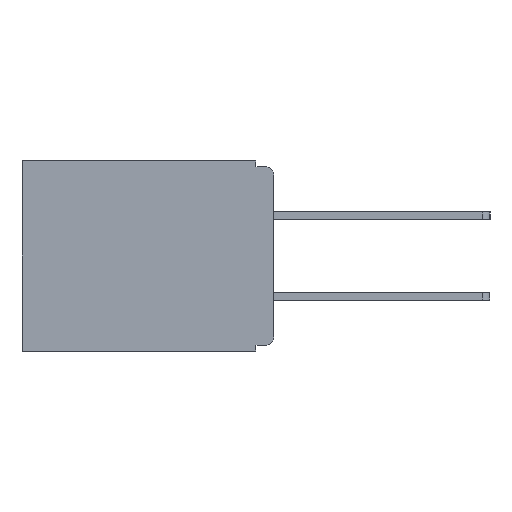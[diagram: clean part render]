
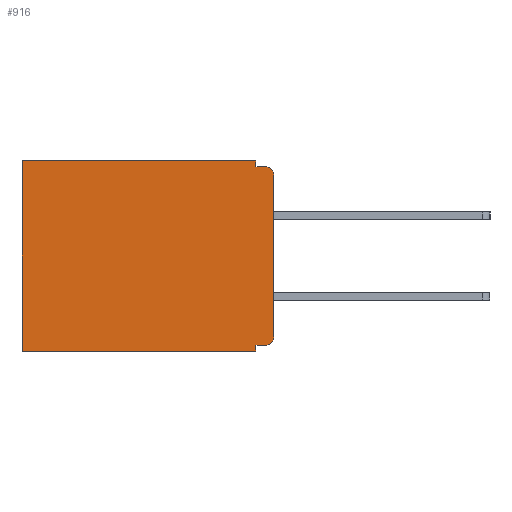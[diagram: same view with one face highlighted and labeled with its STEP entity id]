
A CAD part, left-side view. The second image highlights one B-rep face of the part: STEP entity #916.
In plain terms, the highlighted planar face has unit normal (-1, 0, 0).
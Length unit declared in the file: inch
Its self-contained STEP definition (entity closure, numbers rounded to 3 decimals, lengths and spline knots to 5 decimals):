
#257 = EDGE_CURVE ( 'NONE', #17547, #11450, #16624, .T. ) ;
#295 = CARTESIAN_POINT ( 'NONE',  ( 0.3, 0., -0.305 ) ) ;
#729 = EDGE_CURVE ( 'NONE', #16761, #9705, #21388, .T. ) ;
#916 = ADVANCED_FACE ( 'NONE', ( #12551 ), #16678, .F. ) ;
#1194 = DIRECTION ( 'NONE',  ( 1., 0., 0. ) ) ;
#1379 = EDGE_CURVE ( 'NONE', #1905, #20736, #11943, .T. ) ;
#1408 = LINE ( 'NONE', #9145, #15512 ) ;
#1905 = VERTEX_POINT ( 'NONE', #21565 ) ;
#1926 = VERTEX_POINT ( 'NONE', #21072 ) ;
#1975 = VECTOR ( 'NONE', #15473, 39.37008 ) ;
#2044 = VERTEX_POINT ( 'NONE', #295 ) ;
#2664 = CIRCLE ( 'NONE', #19010, 0.015 ) ;
#3220 = ORIENTED_EDGE ( 'NONE', *, *, #19038, .T. ) ;
#3266 = VECTOR ( 'NONE', #14020, 39.37008 ) ;
#3388 = DIRECTION ( 'NONE',  ( 0., 0., -1. ) ) ;
#5273 = ORIENTED_EDGE ( 'NONE', *, *, #23190, .T. ) ;
#6233 = CARTESIAN_POINT ( 'NONE',  ( 0.3, 0., -0.025 ) ) ;
#6611 = ORIENTED_EDGE ( 'NONE', *, *, #7758, .F. ) ;
#6916 = VECTOR ( 'NONE', #12707, 39.37008 ) ;
#7016 = CARTESIAN_POINT ( 'NONE',  ( 0.3, 0.031, -0.33 ) ) ;
#7121 = CARTESIAN_POINT ( 'NONE',  ( 0.3, 0.031, -0.32 ) ) ;
#7141 = CARTESIAN_POINT ( 'NONE',  ( 0.3, 0., -0.33 ) ) ;
#7564 = CARTESIAN_POINT ( 'NONE',  ( 0.3, 0., -0.33 ) ) ;
#7758 = EDGE_CURVE ( 'NONE', #20229, #9705, #18964, .T. ) ;
#8225 = CARTESIAN_POINT ( 'NONE',  ( 0.3, 0.015, -0.025 ) ) ;
#8799 = EDGE_CURVE ( 'NONE', #11450, #1926, #1408, .T. ) ;
#8813 = DIRECTION ( 'NONE',  ( 0., 0., -1. ) ) ;
#8889 = ORIENTED_EDGE ( 'NONE', *, *, #1379, .F. ) ;
#9055 = VERTEX_POINT ( 'NONE', #6233 ) ;
#9145 = CARTESIAN_POINT ( 'NONE',  ( 0.3, 0., -0.01 ) ) ;
#9475 = CARTESIAN_POINT ( 'NONE',  ( 0.3, 0.015, -0.305 ) ) ;
#9705 = VERTEX_POINT ( 'NONE', #13514 ) ;
#9715 = LINE ( 'NONE', #7016, #14582 ) ;
#10047 = DIRECTION ( 'NONE',  ( 0., 0., -1. ) ) ;
#10488 = CARTESIAN_POINT ( 'NONE',  ( 0.3, 0.437, -0.33 ) ) ;
#10708 = CARTESIAN_POINT ( 'NONE',  ( 0.3, 0., -0.33 ) ) ;
#11182 = CARTESIAN_POINT ( 'NONE',  ( 0.3, 0.031, 0. ) ) ;
#11273 = DIRECTION ( 'NONE',  ( 0., 0., -1. ) ) ;
#11450 = VERTEX_POINT ( 'NONE', #22516 ) ;
#11943 = LINE ( 'NONE', #19986, #16837 ) ;
#12072 = CARTESIAN_POINT ( 'NONE',  ( 0.3, 0., 0. ) ) ;
#12343 = ORIENTED_EDGE ( 'NONE', *, *, #257, .F. ) ;
#12551 = FACE_OUTER_BOUND ( 'NONE', #17389, .T. ) ;
#12707 = DIRECTION ( 'NONE',  ( 0., 0., -1. ) ) ;
#12970 = ORIENTED_EDGE ( 'NONE', *, *, #22609, .T. ) ;
#13514 = CARTESIAN_POINT ( 'NONE',  ( 0.3, 0.437, -0.33 ) ) ;
#13988 = CARTESIAN_POINT ( 'NONE',  ( 0.3, 0.031, 0. ) ) ;
#14020 = DIRECTION ( 'NONE',  ( 0., 1., 0. ) ) ;
#14120 = VECTOR ( 'NONE', #22031, 39.37008 ) ;
#14582 = VECTOR ( 'NONE', #8813, 39.37008 ) ;
#14674 = DIRECTION ( 'NONE',  ( 0., -1., 0. ) ) ;
#14936 = CARTESIAN_POINT ( 'NONE',  ( 0.3, 0.031, -0.33 ) ) ;
#15131 = CIRCLE ( 'NONE', #22781, 0.015 ) ;
#15473 = DIRECTION ( 'NONE',  ( 0., 0., -1. ) ) ;
#15512 = VECTOR ( 'NONE', #14674, 39.37008 ) ;
#15658 = LINE ( 'NONE', #10708, #19895 ) ;
#16264 = CARTESIAN_POINT ( 'NONE',  ( 0.3, 0.437, 0. ) ) ;
#16624 = LINE ( 'NONE', #13988, #1975 ) ;
#16678 = PLANE ( 'NONE',  #21882 ) ;
#16761 = VERTEX_POINT ( 'NONE', #16264 ) ;
#16837 = VECTOR ( 'NONE', #19875, 39.37008 ) ;
#17375 = EDGE_CURVE ( 'NONE', #9055, #2044, #15658, .T. ) ;
#17389 = EDGE_LOOP ( 'NONE', ( #21274, #12970, #17854, #12343, #5273, #21828, #6611, #18750, #8889, #3220 ) ) ;
#17547 = VERTEX_POINT ( 'NONE', #11182 ) ;
#17854 = ORIENTED_EDGE ( 'NONE', *, *, #8799, .F. ) ;
#18750 = ORIENTED_EDGE ( 'NONE', *, *, #21571, .F. ) ;
#18964 = LINE ( 'NONE', #7564, #14120 ) ;
#19010 = AXIS2_PLACEMENT_3D ( 'NONE', #9475, #22148, #11273 ) ;
#19038 = EDGE_CURVE ( 'NONE', #1905, #2044, #2664, .T. ) ;
#19875 = DIRECTION ( 'NONE',  ( 0., 1., 0. ) ) ;
#19895 = VECTOR ( 'NONE', #21596, 39.37008 ) ;
#19986 = CARTESIAN_POINT ( 'NONE',  ( 0.3, 0., -0.32 ) ) ;
#20229 = VERTEX_POINT ( 'NONE', #14936 ) ;
#20736 = VERTEX_POINT ( 'NONE', #7121 ) ;
#20950 = DIRECTION ( 'NONE',  ( -1., 0., 0. ) ) ;
#21072 = CARTESIAN_POINT ( 'NONE',  ( 0.3, 0.015, -0.01 ) ) ;
#21274 = ORIENTED_EDGE ( 'NONE', *, *, #17375, .F. ) ;
#21388 = LINE ( 'NONE', #10488, #6916 ) ;
#21565 = CARTESIAN_POINT ( 'NONE',  ( 0.3, 0.015, -0.32 ) ) ;
#21571 = EDGE_CURVE ( 'NONE', #20736, #20229, #9715, .T. ) ;
#21596 = DIRECTION ( 'NONE',  ( 0., 0., -1. ) ) ;
#21828 = ORIENTED_EDGE ( 'NONE', *, *, #729, .T. ) ;
#21882 = AXIS2_PLACEMENT_3D ( 'NONE', #7141, #1194, #3388 ) ;
#22031 = DIRECTION ( 'NONE',  ( 0., 1., 0. ) ) ;
#22148 = DIRECTION ( 'NONE',  ( -1., 0., 0. ) ) ;
#22516 = CARTESIAN_POINT ( 'NONE',  ( 0.3, 0.031, -0.01 ) ) ;
#22597 = LINE ( 'NONE', #12072, #3266 ) ;
#22609 = EDGE_CURVE ( 'NONE', #9055, #1926, #15131, .T. ) ;
#22781 = AXIS2_PLACEMENT_3D ( 'NONE', #8225, #20950, #10047 ) ;
#23190 = EDGE_CURVE ( 'NONE', #17547, #16761, #22597, .T. ) ;
